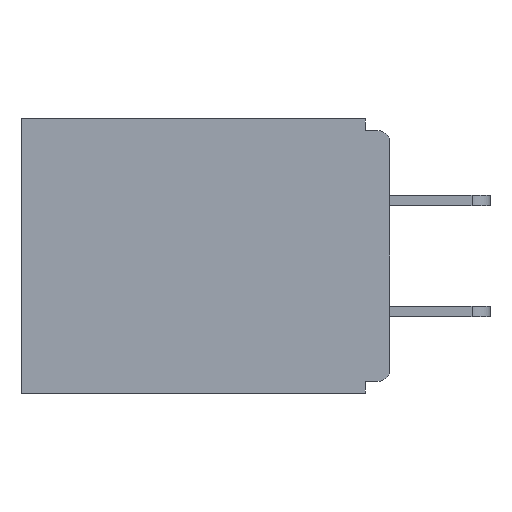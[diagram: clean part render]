
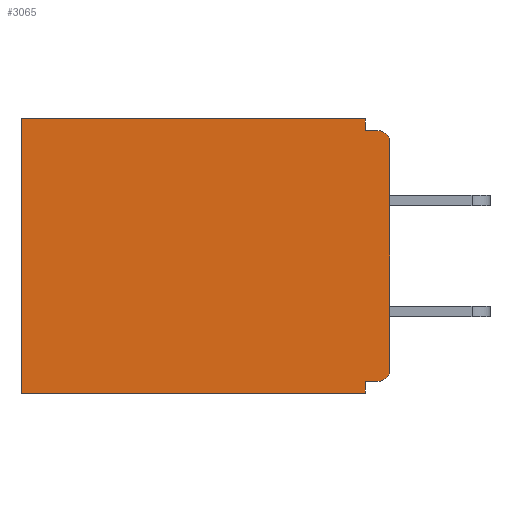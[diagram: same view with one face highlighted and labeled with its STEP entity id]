
A CAD part, left-side view. The second image highlights one B-rep face of the part: STEP entity #3065.
In plain terms, the highlighted planar face has unit normal (-1, 0, 0).
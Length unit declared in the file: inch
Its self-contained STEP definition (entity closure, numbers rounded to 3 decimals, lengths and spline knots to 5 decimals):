
#31 = EDGE_CURVE ( 'NONE', #2447, #2945, #8577, .T. ) ;
#377 = CARTESIAN_POINT ( 'NONE',  ( 0.298, 0.46, 0. ) ) ;
#578 = DIRECTION ( 'NONE',  ( 0., 0., -1. ) ) ;
#637 = VECTOR ( 'NONE', #4130, 39.37008 ) ;
#689 = ORIENTED_EDGE ( 'NONE', *, *, #4553, .T. ) ;
#918 = VECTOR ( 'NONE', #1971, 39.37008 ) ;
#1047 = DIRECTION ( 'NONE',  ( 0., 0., -1. ) ) ;
#1127 = PLANE ( 'NONE',  #4615 ) ;
#1144 = LINE ( 'NONE', #11124, #5811 ) ;
#1261 = VECTOR ( 'NONE', #8907, 39.37008 ) ;
#1922 = ORIENTED_EDGE ( 'NONE', *, *, #9953, .T. ) ;
#1971 = DIRECTION ( 'NONE',  ( 0., 1., 0. ) ) ;
#2085 = ORIENTED_EDGE ( 'NONE', *, *, #5377, .T. ) ;
#2289 = CARTESIAN_POINT ( 'NONE',  ( 0.298, 0.031, -0.015 ) ) ;
#2370 = CARTESIAN_POINT ( 'NONE',  ( 0.298, 0.031, -0.328 ) ) ;
#2447 = VERTEX_POINT ( 'NONE', #6541 ) ;
#2537 = DIRECTION ( 'NONE',  ( -1., 0., 0. ) ) ;
#2717 = VERTEX_POINT ( 'NONE', #2289 ) ;
#2945 = VERTEX_POINT ( 'NONE', #8539 ) ;
#3015 = CARTESIAN_POINT ( 'NONE',  ( 0.298, 0.46, 0. ) ) ;
#3065 = ADVANCED_FACE ( 'NONE', ( #11245 ), #1127, .F. ) ;
#3195 = AXIS2_PLACEMENT_3D ( 'NONE', #8252, #6282, #578 ) ;
#3310 = VERTEX_POINT ( 'NONE', #2370 ) ;
#3313 = EDGE_CURVE ( 'NONE', #3310, #2447, #6001, .T. ) ;
#3425 = VERTEX_POINT ( 'NONE', #377 ) ;
#3445 = CARTESIAN_POINT ( 'NONE',  ( 0.298, 0., -0.328 ) ) ;
#3851 = VERTEX_POINT ( 'NONE', #5972 ) ;
#3996 = ORIENTED_EDGE ( 'NONE', *, *, #3313, .F. ) ;
#4024 = CARTESIAN_POINT ( 'NONE',  ( 0.298, 0., 0. ) ) ;
#4107 = ORIENTED_EDGE ( 'NONE', *, *, #8838, .F. ) ;
#4116 = CIRCLE ( 'NONE', #5736, 0.015 ) ;
#4130 = DIRECTION ( 'NONE',  ( 0., -1., 0. ) ) ;
#4133 = ORIENTED_EDGE ( 'NONE', *, *, #9315, .F. ) ;
#4157 = LINE ( 'NONE', #3445, #5968 ) ;
#4389 = VECTOR ( 'NONE', #8486, 39.37008 ) ;
#4553 = EDGE_CURVE ( 'NONE', #8310, #5650, #5950, .T. ) ;
#4615 = AXIS2_PLACEMENT_3D ( 'NONE', #9745, #6791, #1047 ) ;
#4878 = ORIENTED_EDGE ( 'NONE', *, *, #6109, .F. ) ;
#5377 = EDGE_CURVE ( 'NONE', #3425, #2945, #6061, .T. ) ;
#5650 = VERTEX_POINT ( 'NONE', #12213 ) ;
#5736 = AXIS2_PLACEMENT_3D ( 'NONE', #9229, #2537, #11173 ) ;
#5811 = VECTOR ( 'NONE', #12081, 39.37008 ) ;
#5950 = CIRCLE ( 'NONE', #3195, 0.015 ) ;
#5968 = VECTOR ( 'NONE', #10186, 39.37008 ) ;
#5972 = CARTESIAN_POINT ( 'NONE',  ( 0.298, 0.015, -0.328 ) ) ;
#6001 = LINE ( 'NONE', #6267, #12125 ) ;
#6061 = LINE ( 'NONE', #3015, #8333 ) ;
#6109 = EDGE_CURVE ( 'NONE', #2717, #5650, #6310, .T. ) ;
#6267 = CARTESIAN_POINT ( 'NONE',  ( 0.298, 0.031, -0.343 ) ) ;
#6282 = DIRECTION ( 'NONE',  ( -1., 0., 0. ) ) ;
#6310 = LINE ( 'NONE', #11796, #637 ) ;
#6541 = CARTESIAN_POINT ( 'NONE',  ( 0.298, 0.031, -0.343 ) ) ;
#6791 = DIRECTION ( 'NONE',  ( 1., 0., 0. ) ) ;
#6800 = CARTESIAN_POINT ( 'NONE',  ( 0.298, 0., -0.313 ) ) ;
#7427 = ORIENTED_EDGE ( 'NONE', *, *, #11323, .F. ) ;
#7527 = CARTESIAN_POINT ( 'NONE',  ( 0.298, 0.031, -0.343 ) ) ;
#7819 = VERTEX_POINT ( 'NONE', #6800 ) ;
#7890 = EDGE_LOOP ( 'NONE', ( #689, #4878, #7427, #1922, #2085, #8926, #3996, #4107, #11010, #4133 ) ) ;
#8252 = CARTESIAN_POINT ( 'NONE',  ( 0.298, 0.015, -0.03 ) ) ;
#8310 = VERTEX_POINT ( 'NONE', #11764 ) ;
#8333 = VECTOR ( 'NONE', #8766, 39.37008 ) ;
#8486 = DIRECTION ( 'NONE',  ( 0., 0., -1. ) ) ;
#8539 = CARTESIAN_POINT ( 'NONE',  ( 0.298, 0.46, -0.343 ) ) ;
#8577 = LINE ( 'NONE', #10192, #918 ) ;
#8766 = DIRECTION ( 'NONE',  ( 0., 0., -1. ) ) ;
#8838 = EDGE_CURVE ( 'NONE', #3851, #3310, #4157, .T. ) ;
#8907 = DIRECTION ( 'NONE',  ( 0., 1., 0. ) ) ;
#8926 = ORIENTED_EDGE ( 'NONE', *, *, #31, .F. ) ;
#9229 = CARTESIAN_POINT ( 'NONE',  ( 0.298, 0.015, -0.313 ) ) ;
#9315 = EDGE_CURVE ( 'NONE', #8310, #7819, #1144, .T. ) ;
#9634 = CARTESIAN_POINT ( 'NONE',  ( 0.298, 0.031, 0. ) ) ;
#9745 = CARTESIAN_POINT ( 'NONE',  ( 0.298, 0., 0. ) ) ;
#9953 = EDGE_CURVE ( 'NONE', #11887, #3425, #11019, .T. ) ;
#10186 = DIRECTION ( 'NONE',  ( 0., 1., 0. ) ) ;
#10192 = CARTESIAN_POINT ( 'NONE',  ( 0.298, 0., -0.343 ) ) ;
#10671 = EDGE_CURVE ( 'NONE', #3851, #7819, #4116, .T. ) ;
#11010 = ORIENTED_EDGE ( 'NONE', *, *, #10671, .T. ) ;
#11019 = LINE ( 'NONE', #4024, #1261 ) ;
#11124 = CARTESIAN_POINT ( 'NONE',  ( 0.298, 0., 0. ) ) ;
#11173 = DIRECTION ( 'NONE',  ( 0., 0., -1. ) ) ;
#11245 = FACE_OUTER_BOUND ( 'NONE', #7890, .T. ) ;
#11323 = EDGE_CURVE ( 'NONE', #11887, #2717, #11889, .T. ) ;
#11764 = CARTESIAN_POINT ( 'NONE',  ( 0.298, 0., -0.03 ) ) ;
#11796 = CARTESIAN_POINT ( 'NONE',  ( 0.298, 0., -0.015 ) ) ;
#11887 = VERTEX_POINT ( 'NONE', #9634 ) ;
#11889 = LINE ( 'NONE', #7527, #4389 ) ;
#11970 = DIRECTION ( 'NONE',  ( 0., 0., -1. ) ) ;
#12081 = DIRECTION ( 'NONE',  ( 0., 0., -1. ) ) ;
#12125 = VECTOR ( 'NONE', #11970, 39.37008 ) ;
#12213 = CARTESIAN_POINT ( 'NONE',  ( 0.298, 0.015, -0.015 ) ) ;
